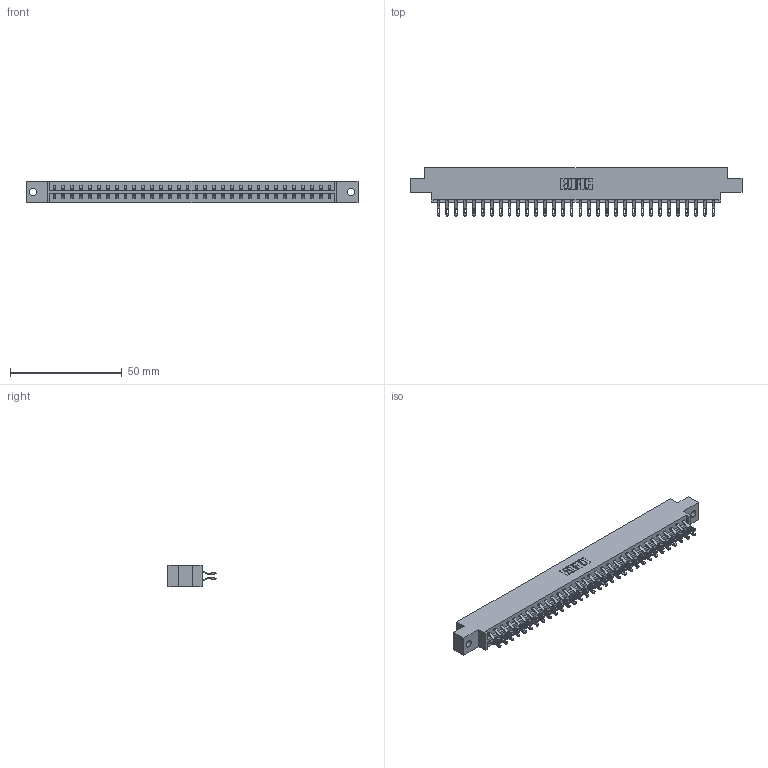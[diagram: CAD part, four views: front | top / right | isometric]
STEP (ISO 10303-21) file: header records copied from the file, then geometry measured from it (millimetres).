
FILE_DESCRIPTION (( 'STEP AP203' ), '1' );
FILE_NAME ('833-064-555-802.STEP', '2020-06-05T07:41:02', ( '' ), ( '' ), 'SwSTEP 2.0', 'SolidWorks 2020', '' );
FILE_SCHEMA (( 'CONFIG_CONTROL_DESIGN' ));
Length unit declared in the file: inch
Products named in the file (3): 833 Part_Offset - .128 Dia; 833-064-555-802; 345-292-001_555 Tail
Assembly tree (65 placements, depth 2):
  833-064-555-802
    833 Part_Offset - .128 Dia
    345-292-001_555 Tail  x64
Bounding box: 148.34 x 21.47 x 9.4 mm (x, y, z)
Volume: 14971.9 mm3; surface area: 18234.8 mm2
Topology: 65 solids, 65 shells, 3830 faces, 12035 edges, 8022 vertices
Faces by surface type: plane 2250, cylinder 1580
Entity records: 22341 total; most frequent: CARTESIAN_POINT 3752, ORIENTED_EDGE 3658, DIRECTION 3193, EDGE_CURVE 1829, VECTOR 1681, LINE 1681, VERTEX_POINT 1218, AXIS2_PLACEMENT_3D 756
